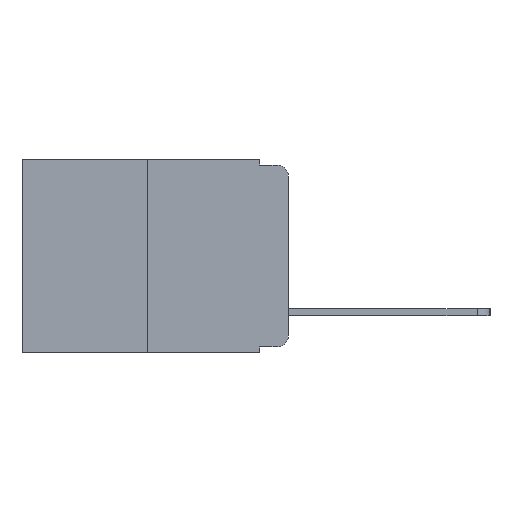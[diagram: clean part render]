
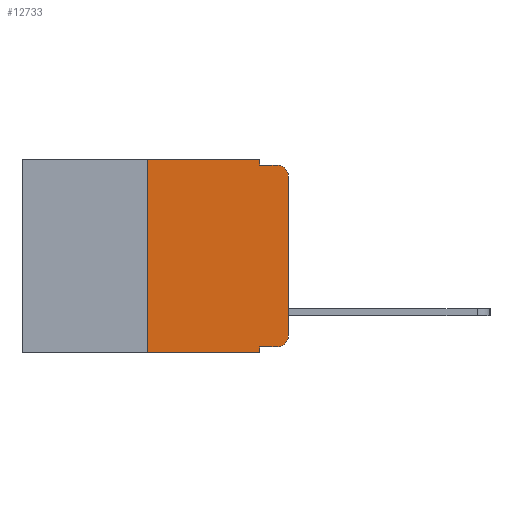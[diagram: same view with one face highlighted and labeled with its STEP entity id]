
A CAD part, left-side view. The second image highlights one B-rep face of the part: STEP entity #12733.
In plain terms, the highlighted planar face has unit normal (-1, 0, 0).
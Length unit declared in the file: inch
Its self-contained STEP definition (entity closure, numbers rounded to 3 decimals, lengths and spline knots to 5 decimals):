
#160 = VERTEX_POINT ( 'NONE', #9760 ) ;
#211 = CARTESIAN_POINT ( 'NONE',  ( 0., 0.02, -0.333 ) ) ;
#557 = CARTESIAN_POINT ( 'NONE',  ( 0., 0., 0. ) ) ;
#744 = LINE ( 'NONE', #4139, #11409 ) ;
#773 = EDGE_CURVE ( 'NONE', #6534, #17053, #6641, .T. ) ;
#1703 = DIRECTION ( 'NONE',  ( 0., -1., 0. ) ) ;
#2091 = VECTOR ( 'NONE', #12177, 39.37008 ) ;
#2172 = AXIS2_PLACEMENT_3D ( 'NONE', #16692, #7926, #18153 ) ;
#2528 = EDGE_CURVE ( 'NONE', #14765, #6606, #5148, .T. ) ;
#2613 = VERTEX_POINT ( 'NONE', #11006 ) ;
#2885 = ORIENTED_EDGE ( 'NONE', *, *, #5350, .T. ) ;
#3227 = CARTESIAN_POINT ( 'NONE',  ( 0., 0.473, -0.343 ) ) ;
#3376 = CARTESIAN_POINT ( 'NONE',  ( 0., 0.02, -0.03 ) ) ;
#3870 = CARTESIAN_POINT ( 'NONE',  ( 0., 0.25, 0. ) ) ;
#4003 = LINE ( 'NONE', #9275, #15352 ) ;
#4139 = CARTESIAN_POINT ( 'NONE',  ( 0., 0.051, -0.333 ) ) ;
#4309 = LINE ( 'NONE', #15752, #15625 ) ;
#4563 = EDGE_LOOP ( 'NONE', ( #8593, #5809, #15902, #15934, #11087, #5331, #11663, #15074, #2885, #16150 ) ) ;
#4584 = EDGE_CURVE ( 'NONE', #2613, #6534, #4003, .T. ) ;
#4872 = CARTESIAN_POINT ( 'NONE',  ( 0., 0.051, 0. ) ) ;
#4908 = DIRECTION ( 'NONE',  ( 0., 0., -1. ) ) ;
#5148 = CIRCLE ( 'NONE', #11695, 0.02 ) ;
#5331 = ORIENTED_EDGE ( 'NONE', *, *, #15251, .F. ) ;
#5350 = EDGE_CURVE ( 'NONE', #19206, #12359, #744, .T. ) ;
#5724 = CARTESIAN_POINT ( 'NONE',  ( 0., 0.473, 0. ) ) ;
#5808 = CARTESIAN_POINT ( 'NONE',  ( 0., 0.051, -0.333 ) ) ;
#5809 = ORIENTED_EDGE ( 'NONE', *, *, #2528, .T. ) ;
#5990 = EDGE_CURVE ( 'NONE', #17053, #6606, #4309, .T. ) ;
#6131 = CARTESIAN_POINT ( 'NONE',  ( 0., 0.051, -0.01 ) ) ;
#6534 = VERTEX_POINT ( 'NONE', #11144 ) ;
#6606 = VERTEX_POINT ( 'NONE', #11323 ) ;
#6641 = LINE ( 'NONE', #16361, #18762 ) ;
#6659 = VECTOR ( 'NONE', #11179, 39.37008 ) ;
#6959 = DIRECTION ( 'NONE',  ( 0., -1., 0. ) ) ;
#7012 = EDGE_CURVE ( 'NONE', #17242, #160, #7110, .T. ) ;
#7110 = LINE ( 'NONE', #3227, #2091 ) ;
#7275 = PLANE ( 'NONE',  #14540 ) ;
#7397 = FACE_OUTER_BOUND ( 'NONE', #4563, .T. ) ;
#7926 = DIRECTION ( 'NONE',  ( -1., 0., 0. ) ) ;
#8028 = CARTESIAN_POINT ( 'NONE',  ( 0., 0.25, -0.343 ) ) ;
#8593 = ORIENTED_EDGE ( 'NONE', *, *, #14527, .T. ) ;
#8790 = DIRECTION ( 'NONE',  ( 0., 0., -1. ) ) ;
#9275 = CARTESIAN_POINT ( 'NONE',  ( 0., 0.473, 0. ) ) ;
#9760 = CARTESIAN_POINT ( 'NONE',  ( 0., 0.051, -0.343 ) ) ;
#10198 = CARTESIAN_POINT ( 'NONE',  ( 0., 0., -0.03 ) ) ;
#10340 = CIRCLE ( 'NONE', #2172, 0.02 ) ;
#10682 = VECTOR ( 'NONE', #14248, 39.37008 ) ;
#11006 = CARTESIAN_POINT ( 'NONE',  ( 0., 0.25, 0. ) ) ;
#11087 = ORIENTED_EDGE ( 'NONE', *, *, #4584, .F. ) ;
#11144 = CARTESIAN_POINT ( 'NONE',  ( 0., 0.051, 0. ) ) ;
#11179 = DIRECTION ( 'NONE',  ( 0., 0., 1. ) ) ;
#11323 = CARTESIAN_POINT ( 'NONE',  ( 0., 0.02, -0.01 ) ) ;
#11409 = VECTOR ( 'NONE', #13053, 39.37008 ) ;
#11663 = ORIENTED_EDGE ( 'NONE', *, *, #7012, .T. ) ;
#11695 = AXIS2_PLACEMENT_3D ( 'NONE', #3376, #13800, #4908 ) ;
#11749 = DIRECTION ( 'NONE',  ( 0., 0., -1. ) ) ;
#12177 = DIRECTION ( 'NONE',  ( 0., -1., 0. ) ) ;
#12202 = CARTESIAN_POINT ( 'NONE',  ( 0., 0., -0.313 ) ) ;
#12327 = EDGE_CURVE ( 'NONE', #19206, #160, #13442, .T. ) ;
#12359 = VERTEX_POINT ( 'NONE', #211 ) ;
#12733 = ADVANCED_FACE ( 'NONE', ( #7397 ), #7275, .F. ) ;
#12990 = VERTEX_POINT ( 'NONE', #12202 ) ;
#13053 = DIRECTION ( 'NONE',  ( 0., -1., 0. ) ) ;
#13442 = LINE ( 'NONE', #4872, #17270 ) ;
#13800 = DIRECTION ( 'NONE',  ( -1., 0., 0. ) ) ;
#14248 = DIRECTION ( 'NONE',  ( 0., 0., 1. ) ) ;
#14527 = EDGE_CURVE ( 'NONE', #12990, #14765, #18340, .T. ) ;
#14540 = AXIS2_PLACEMENT_3D ( 'NONE', #5724, #17534, #8790 ) ;
#14765 = VERTEX_POINT ( 'NONE', #10198 ) ;
#15074 = ORIENTED_EDGE ( 'NONE', *, *, #12327, .F. ) ;
#15251 = EDGE_CURVE ( 'NONE', #17242, #2613, #17982, .T. ) ;
#15352 = VECTOR ( 'NONE', #1703, 39.37008 ) ;
#15625 = VECTOR ( 'NONE', #6959, 39.37008 ) ;
#15752 = CARTESIAN_POINT ( 'NONE',  ( 0., 0.051, -0.01 ) ) ;
#15902 = ORIENTED_EDGE ( 'NONE', *, *, #5990, .F. ) ;
#15934 = ORIENTED_EDGE ( 'NONE', *, *, #773, .F. ) ;
#16150 = ORIENTED_EDGE ( 'NONE', *, *, #18358, .T. ) ;
#16361 = CARTESIAN_POINT ( 'NONE',  ( 0., 0.051, 0. ) ) ;
#16692 = CARTESIAN_POINT ( 'NONE',  ( 0., 0.02, -0.313 ) ) ;
#17053 = VERTEX_POINT ( 'NONE', #6131 ) ;
#17242 = VERTEX_POINT ( 'NONE', #8028 ) ;
#17270 = VECTOR ( 'NONE', #18125, 39.37008 ) ;
#17534 = DIRECTION ( 'NONE',  ( 1., 0., 0. ) ) ;
#17982 = LINE ( 'NONE', #3870, #10682 ) ;
#18125 = DIRECTION ( 'NONE',  ( 0., 0., -1. ) ) ;
#18153 = DIRECTION ( 'NONE',  ( 0., 0., -1. ) ) ;
#18340 = LINE ( 'NONE', #557, #6659 ) ;
#18358 = EDGE_CURVE ( 'NONE', #12359, #12990, #10340, .T. ) ;
#18762 = VECTOR ( 'NONE', #11749, 39.37008 ) ;
#19206 = VERTEX_POINT ( 'NONE', #5808 ) ;
